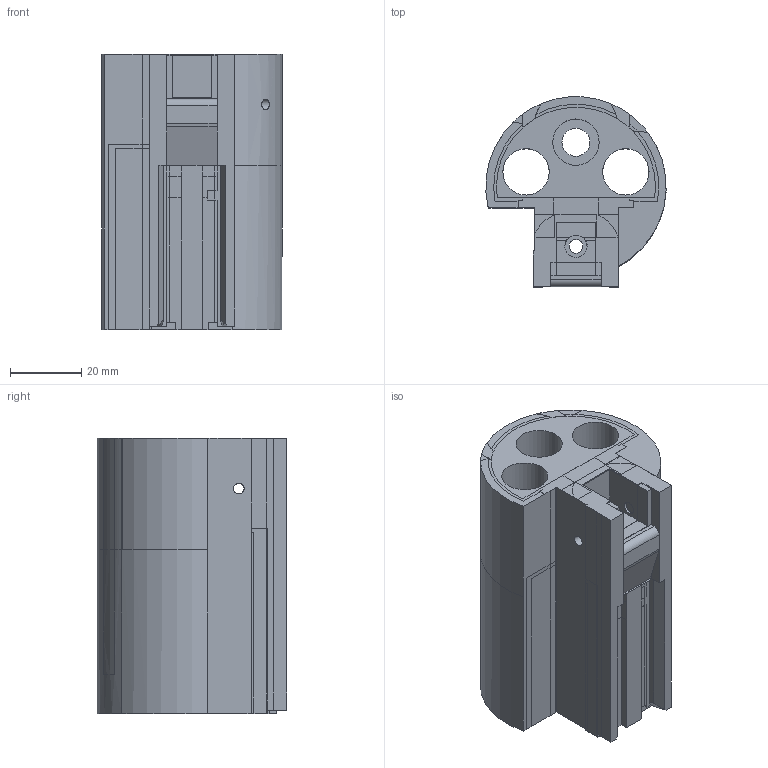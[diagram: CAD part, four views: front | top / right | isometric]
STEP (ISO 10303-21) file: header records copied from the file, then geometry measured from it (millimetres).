
FILE_DESCRIPTION(('FreeCAD Model'),'2;1');
FILE_NAME('mp-1 bolt housing.step','2016-03-27T02:54:47',('Author'),(''), 'Open CASCADE STEP processor 6.8','FreeCAD','Unknown');
FILE_SCHEMA(('AUTOMOTIVE_DESIGN_CC2 { 1 2 10303 214 -1 1 5 4 }'));
Length unit declared in the file: millimetre
Products named in the file (1): Pocket013
Bounding box: 50.53 x 53.27 x 77.2 mm (x, y, z)
Volume: 64152.2 mm3; surface area: 29408.5 mm2
Topology: 1 solids, 1 shells, 253 faces, 725 edges, 478 vertices
Faces by surface type: plane 196, cylinder 56, extrusion 1
Full cylindrical faces by diameter (mm): 3 x1, 3.566 x1, 3.861 x1, 6.25 x1, 7.85 x1, 13 x3
Entity records: 20974 total; most frequent: CARTESIAN_POINT 7198, DIRECTION 2361, VECTOR 1561, LINE 1560, ORIENTED_EDGE 1450, PCURVE 1450, DEFINITIONAL_REPRESENTATION 1450, EDGE_CURVE 725
